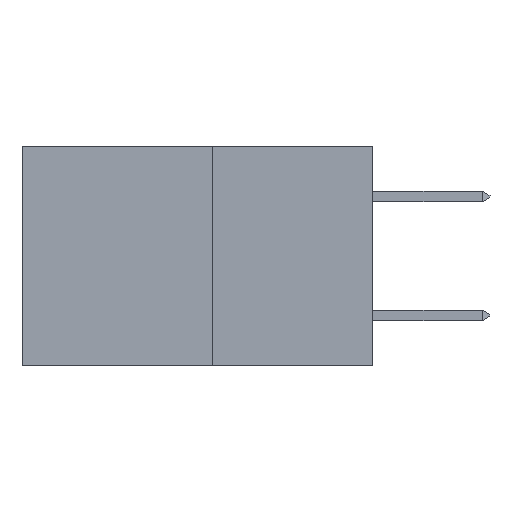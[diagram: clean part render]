
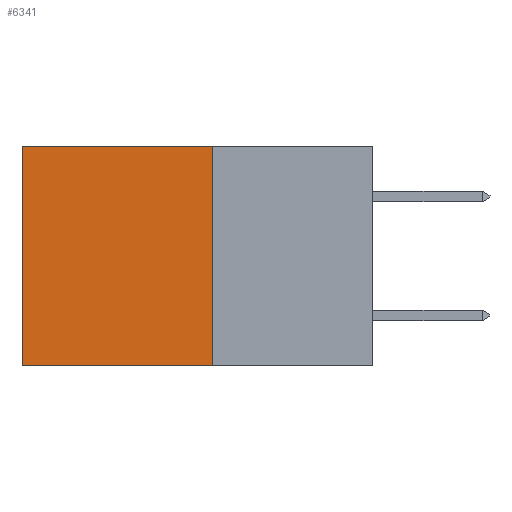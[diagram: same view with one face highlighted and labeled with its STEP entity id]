
A CAD part, left-side view. The second image highlights one B-rep face of the part: STEP entity #6341.
In plain terms, the highlighted planar face has unit normal (-1, 0, 0).
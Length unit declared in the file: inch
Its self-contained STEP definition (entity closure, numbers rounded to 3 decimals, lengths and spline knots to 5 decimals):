
#181 = DIRECTION ( 'NONE',  ( 0., 0., -1. ) ) ;
#201 = DIRECTION ( 'NONE',  ( 1., 0., 0. ) ) ;
#224 = PLANE ( 'NONE',  #6197 ) ;
#305 = CARTESIAN_POINT ( 'NONE',  ( 0.277, 0.27, -0.37 ) ) ;
#517 = VERTEX_POINT ( 'NONE', #6151 ) ;
#661 = DIRECTION ( 'NONE',  ( 0., 1., 0. ) ) ;
#671 = CARTESIAN_POINT ( 'NONE',  ( 0.277, 0.27, 0. ) ) ;
#737 = CARTESIAN_POINT ( 'NONE',  ( 0.277, 0.27, 0. ) ) ;
#804 = VECTOR ( 'NONE', #4201, 39.37008 ) ;
#1991 = VECTOR ( 'NONE', #661, 39.37008 ) ;
#2613 = VECTOR ( 'NONE', #6714, 39.37008 ) ;
#2685 = LINE ( 'NONE', #4536, #804 ) ;
#3012 = EDGE_LOOP ( 'NONE', ( #4812, #5087, #5203, #5818 ) ) ;
#4128 = LINE ( 'NONE', #5770, #7311 ) ;
#4163 = VERTEX_POINT ( 'NONE', #7932 ) ;
#4178 = VERTEX_POINT ( 'NONE', #737 ) ;
#4201 = DIRECTION ( 'NONE',  ( 0., 0., -1. ) ) ;
#4536 = CARTESIAN_POINT ( 'NONE',  ( 0.277, 0.59, -0.37 ) ) ;
#4600 = EDGE_CURVE ( 'NONE', #517, #4163, #6083, .T. ) ;
#4765 = FACE_OUTER_BOUND ( 'NONE', #3012, .T. ) ;
#4812 = ORIENTED_EDGE ( 'NONE', *, *, #6584, .T. ) ;
#5002 = CARTESIAN_POINT ( 'NONE',  ( 0.277, 0.27, -0.37 ) ) ;
#5087 = ORIENTED_EDGE ( 'NONE', *, *, #4600, .F. ) ;
#5203 = ORIENTED_EDGE ( 'NONE', *, *, #7184, .F. ) ;
#5770 = CARTESIAN_POINT ( 'NONE',  ( 0.277, 0.27, -0.37 ) ) ;
#5818 = ORIENTED_EDGE ( 'NONE', *, *, #7869, .T. ) ;
#5827 = DIRECTION ( 'NONE',  ( 0., 0., -1. ) ) ;
#6083 = LINE ( 'NONE', #5002, #2613 ) ;
#6151 = CARTESIAN_POINT ( 'NONE',  ( 0.277, 0.27, -0.37 ) ) ;
#6197 = AXIS2_PLACEMENT_3D ( 'NONE', #305, #201, #181 ) ;
#6341 = ADVANCED_FACE ( 'NONE', ( #4765 ), #224, .F. ) ;
#6381 = VERTEX_POINT ( 'NONE', #8523 ) ;
#6584 = EDGE_CURVE ( 'NONE', #6381, #4163, #2685, .T. ) ;
#6714 = DIRECTION ( 'NONE',  ( 0., 1., 0. ) ) ;
#7184 = EDGE_CURVE ( 'NONE', #4178, #517, #4128, .T. ) ;
#7199 = LINE ( 'NONE', #671, #1991 ) ;
#7311 = VECTOR ( 'NONE', #5827, 39.37008 ) ;
#7869 = EDGE_CURVE ( 'NONE', #4178, #6381, #7199, .T. ) ;
#7932 = CARTESIAN_POINT ( 'NONE',  ( 0.277, 0.59, -0.37 ) ) ;
#8523 = CARTESIAN_POINT ( 'NONE',  ( 0.277, 0.59, 0. ) ) ;
